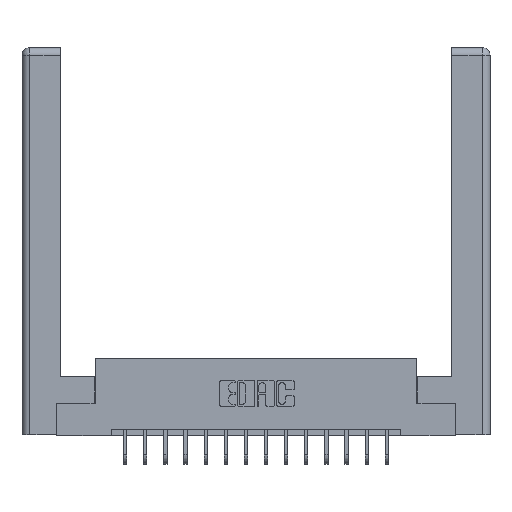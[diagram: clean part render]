
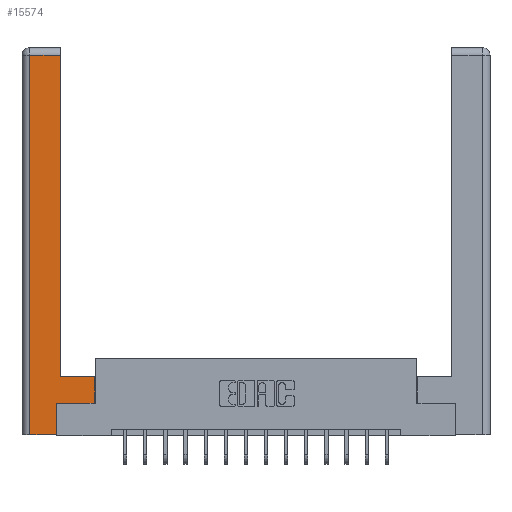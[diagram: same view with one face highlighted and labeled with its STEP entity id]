
A CAD part, top view. The second image highlights one B-rep face of the part: STEP entity #15574.
In plain terms, the highlighted planar face has unit normal (0, 0, 1).
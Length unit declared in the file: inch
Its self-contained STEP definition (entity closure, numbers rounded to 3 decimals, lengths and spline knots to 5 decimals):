
#60 = VERTEX_POINT ( 'NONE', #7357 ) ;
#328 = ORIENTED_EDGE ( 'NONE', *, *, #4388, .T. ) ;
#505 = CARTESIAN_POINT ( 'NONE',  ( 0.265, 0.245, 0. ) ) ;
#587 = LINE ( 'NONE', #11878, #6311 ) ;
#1151 = VERTEX_POINT ( 'NONE', #10224 ) ;
#1236 = EDGE_CURVE ( 'NONE', #11888, #17101, #3767, .T. ) ;
#2275 = PLANE ( 'NONE',  #17366 ) ;
#2629 = EDGE_CURVE ( 'NONE', #17101, #9363, #4850, .T. ) ;
#2855 = VERTEX_POINT ( 'NONE', #13726 ) ;
#2861 = DIRECTION ( 'NONE',  ( -1., 0., 0. ) ) ;
#3256 = DIRECTION ( 'NONE',  ( 1., 0., 0. ) ) ;
#3374 = DIRECTION ( 'NONE',  ( -1., 0., 0. ) ) ;
#3458 = DIRECTION ( 'NONE',  ( 0., 1., 0. ) ) ;
#3563 = CARTESIAN_POINT ( 'NONE',  ( 0., 0., 0. ) ) ;
#3733 = EDGE_CURVE ( 'NONE', #60, #14607, #4334, .T. ) ;
#3767 = LINE ( 'NONE', #505, #6937 ) ;
#4334 = LINE ( 'NONE', #15996, #8875 ) ;
#4338 = LINE ( 'NONE', #5848, #18495 ) ;
#4388 = EDGE_CURVE ( 'NONE', #2855, #1151, #9081, .T. ) ;
#4474 = CARTESIAN_POINT ( 'NONE',  ( 0.295, 0.45, 0. ) ) ;
#4850 = LINE ( 'NONE', #17489, #7805 ) ;
#5848 = CARTESIAN_POINT ( 'NONE',  ( 0.565, 0.45, 0. ) ) ;
#6067 = ORIENTED_EDGE ( 'NONE', *, *, #6631, .T. ) ;
#6251 = VECTOR ( 'NONE', #8645, 39.37008 ) ;
#6311 = VECTOR ( 'NONE', #3256, 39.37008 ) ;
#6631 = EDGE_CURVE ( 'NONE', #12831, #11888, #587, .T. ) ;
#6875 = EDGE_CURVE ( 'NONE', #14607, #2855, #6983, .T. ) ;
#6937 = VECTOR ( 'NONE', #3458, 39.37008 ) ;
#6983 = LINE ( 'NONE', #11328, #18178 ) ;
#7357 = CARTESIAN_POINT ( 'NONE',  ( 0.565, 0.45, 0. ) ) ;
#7805 = VECTOR ( 'NONE', #17559, 39.37008 ) ;
#7813 = ORIENTED_EDGE ( 'NONE', *, *, #13207, .T. ) ;
#7835 = ORIENTED_EDGE ( 'NONE', *, *, #2629, .T. ) ;
#8122 = CARTESIAN_POINT ( 'NONE',  ( 0.0615, 0., 0. ) ) ;
#8594 = CARTESIAN_POINT ( 'NONE',  ( 0.265, 0.245, 0. ) ) ;
#8645 = DIRECTION ( 'NONE',  ( 0., -1., 0. ) ) ;
#8875 = VECTOR ( 'NONE', #2861, 39.37008 ) ;
#9081 = LINE ( 'NONE', #13706, #16392 ) ;
#9111 = FACE_OUTER_BOUND ( 'NONE', #12041, .T. ) ;
#9363 = VERTEX_POINT ( 'NONE', #10672 ) ;
#9977 = ORIENTED_EDGE ( 'NONE', *, *, #1236, .T. ) ;
#10055 = CARTESIAN_POINT ( 'NONE',  ( 0.0615, 0., 0. ) ) ;
#10224 = CARTESIAN_POINT ( 'NONE',  ( 0.0615, 2.94, 0. ) ) ;
#10672 = CARTESIAN_POINT ( 'NONE',  ( 0.565, 0.245, 0. ) ) ;
#10905 = EDGE_CURVE ( 'NONE', #9363, #60, #4338, .T. ) ;
#11328 = CARTESIAN_POINT ( 'NONE',  ( 0.295, 3., 0. ) ) ;
#11878 = CARTESIAN_POINT ( 'NONE',  ( 0.265, 0., 0. ) ) ;
#11888 = VERTEX_POINT ( 'NONE', #15765 ) ;
#12041 = EDGE_LOOP ( 'NONE', ( #15551, #328, #7813, #6067, #9977, #7835, #13874, #17152 ) ) ;
#12432 = DIRECTION ( 'NONE',  ( -1., 0., 0. ) ) ;
#12831 = VERTEX_POINT ( 'NONE', #10055 ) ;
#13207 = EDGE_CURVE ( 'NONE', #1151, #12831, #16511, .T. ) ;
#13706 = CARTESIAN_POINT ( 'NONE',  ( 0.0615, 2.94, 0. ) ) ;
#13726 = CARTESIAN_POINT ( 'NONE',  ( 0.295, 2.94, 0. ) ) ;
#13874 = ORIENTED_EDGE ( 'NONE', *, *, #10905, .T. ) ;
#14558 = DIRECTION ( 'NONE',  ( 0., 1., 0. ) ) ;
#14607 = VERTEX_POINT ( 'NONE', #4474 ) ;
#15551 = ORIENTED_EDGE ( 'NONE', *, *, #6875, .T. ) ;
#15574 = ADVANCED_FACE ( 'NONE', ( #9111 ), #2275, .F. ) ;
#15765 = CARTESIAN_POINT ( 'NONE',  ( 0.265, 0., 0. ) ) ;
#15996 = CARTESIAN_POINT ( 'NONE',  ( 0.295, 0.45, 0. ) ) ;
#16392 = VECTOR ( 'NONE', #3374, 39.37008 ) ;
#16511 = LINE ( 'NONE', #8122, #6251 ) ;
#17101 = VERTEX_POINT ( 'NONE', #8594 ) ;
#17152 = ORIENTED_EDGE ( 'NONE', *, *, #3733, .T. ) ;
#17269 = DIRECTION ( 'NONE',  ( 0., 1., 0. ) ) ;
#17366 = AXIS2_PLACEMENT_3D ( 'NONE', #3563, #18045, #12432 ) ;
#17489 = CARTESIAN_POINT ( 'NONE',  ( 0.565, 0.245, 0. ) ) ;
#17559 = DIRECTION ( 'NONE',  ( 1., 0., 0. ) ) ;
#18045 = DIRECTION ( 'NONE',  ( 0., 0., -1. ) ) ;
#18178 = VECTOR ( 'NONE', #14558, 39.37008 ) ;
#18495 = VECTOR ( 'NONE', #17269, 39.37008 ) ;
